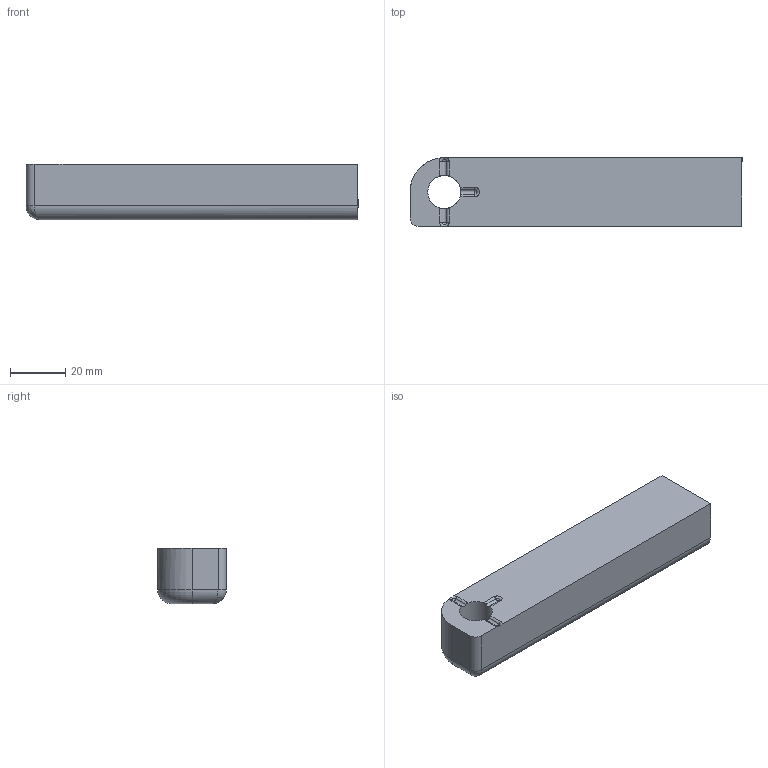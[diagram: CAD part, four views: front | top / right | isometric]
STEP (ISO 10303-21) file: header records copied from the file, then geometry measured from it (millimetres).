
FILE_DESCRIPTION (( 'STEP AP214' ), '1' );
FILE_NAME ('Bipod_Right_Part_2_V2.step', '2016-01-25T18:17:18', ( 'WarFairy' ), ( '' ), 'SwSTEP 2.0', 'SolidWorks 2015', '' );
FILE_SCHEMA (( 'AUTOMOTIVE_DESIGN' ));
Length unit declared in the file: millimetre
Products named in the file (1): Bipod_Right_Part_2_V2
Bounding box: 120 x 24.8 x 20 mm (x, y, z)
Volume: 55111.7 mm3; surface area: 11545.1 mm2
Topology: 1 solids, 1 shells, 45 faces, 130 edges, 73 vertices
Faces by surface type: cylinder 15, sphere 12, torus 10, plane 7, bspline 1
Full cylindrical faces by diameter (mm): 12 x1
Entity records: 1429 total; most frequent: CARTESIAN_POINT 358, DIRECTION 234, ORIENTED_EDGE 208, EDGE_CURVE 104, AXIS2_PLACEMENT_3D 102, VERTEX_POINT 64, CIRCLE 57, EDGE_LOOP 50
